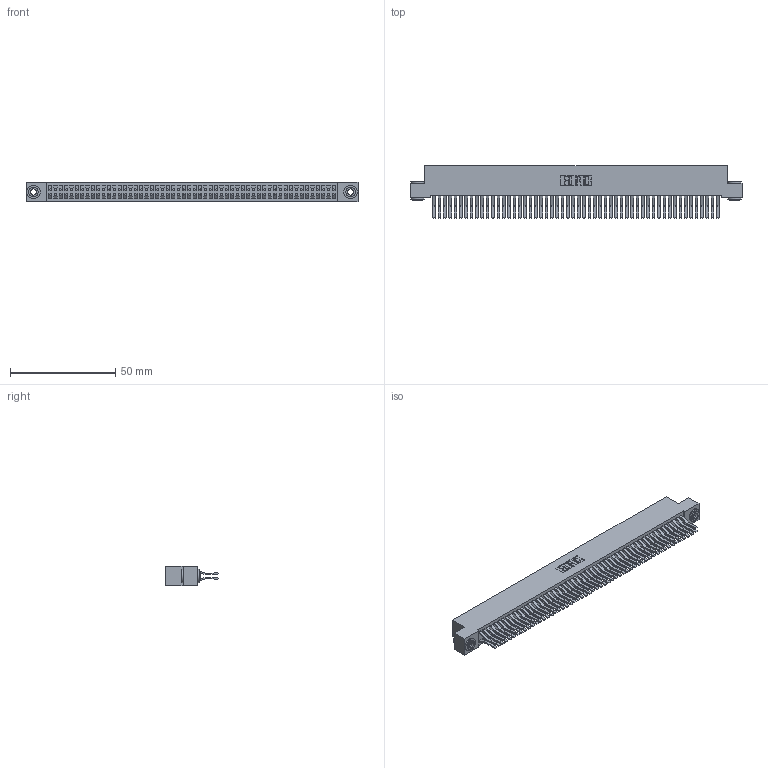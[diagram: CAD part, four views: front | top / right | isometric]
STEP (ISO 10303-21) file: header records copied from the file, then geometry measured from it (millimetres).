
FILE_DESCRIPTION (( 'STEP AP203' ), '1' );
FILE_NAME ('342-108-560-203.STEP', '2019-10-04T20:04:37', ( '' ), ( '' ), 'SwSTEP 2.0', 'SolidWorks 2016', '' );
FILE_SCHEMA (( 'CONFIG_CONTROL_DESIGN' ));
Length unit declared in the file: inch
Products named in the file (4): 342 Part_.156 TH; 345-292-001_560 Tail; 342-250-002_345-250-002-102; 342-108-560-203
Assembly tree (111 placements, depth 2):
  342-108-560-203
    342 Part_.156 TH
    345-292-001_560 Tail  x108
    342-250-002_345-250-002-102  x2
Bounding box: 157.48 x 24.78 x 9.4 mm (x, y, z)
Volume: 14938.2 mm3; surface area: 26525.7 mm2
Topology: 111 solids, 111 shells, 5980 faces, 17763 edges, 11694 vertices
Faces by surface type: plane 3964, cylinder 2008, cone 8
Entity records: 33794 total; most frequent: CARTESIAN_POINT 5561, ORIENTED_EDGE 5490, DIRECTION 4767, EDGE_CURVE 2745, VECTOR 2589, LINE 2589, VERTEX_POINT 1826, AXIS2_PLACEMENT_3D 1089
